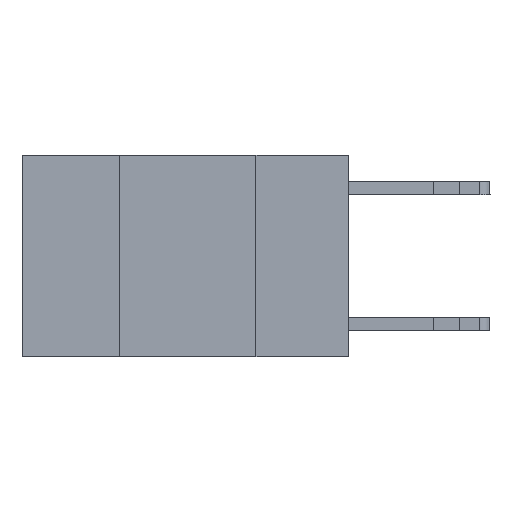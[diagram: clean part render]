
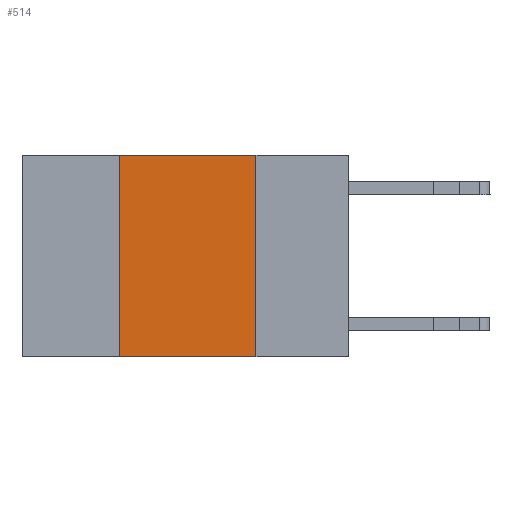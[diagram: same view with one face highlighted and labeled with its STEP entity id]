
A CAD part, left-side view. The second image highlights one B-rep face of the part: STEP entity #514.
In plain terms, the highlighted planar face has unit normal (-1, 0, 0).
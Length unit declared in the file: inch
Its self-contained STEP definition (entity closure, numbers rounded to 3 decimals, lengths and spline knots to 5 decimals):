
#38 = LINE ( 'NONE', #8970, #4514 ) ;
#266 = DIRECTION ( 'NONE',  ( 0., -1., 0. ) ) ;
#419 = EDGE_CURVE ( 'NONE', #13490, #11235, #10476, .T. ) ;
#514 = ADVANCED_FACE ( 'NONE', ( #8455 ), #6282, .F. ) ;
#567 = EDGE_LOOP ( 'NONE', ( #2746, #7116, #1142, #1921 ) ) ;
#623 = CARTESIAN_POINT ( 'NONE',  ( 0., 0.6, -0.37 ) ) ;
#1142 = ORIENTED_EDGE ( 'NONE', *, *, #1852, .F. ) ;
#1598 = AXIS2_PLACEMENT_3D ( 'NONE', #2916, #14141, #8526 ) ;
#1852 = EDGE_CURVE ( 'NONE', #10984, #3160, #9462, .T. ) ;
#1921 = ORIENTED_EDGE ( 'NONE', *, *, #7940, .T. ) ;
#2098 = LINE ( 'NONE', #623, #3636 ) ;
#2198 = CARTESIAN_POINT ( 'NONE',  ( 0., 0.17, 0. ) ) ;
#2746 = ORIENTED_EDGE ( 'NONE', *, *, #419, .F. ) ;
#2916 = CARTESIAN_POINT ( 'NONE',  ( 0., 0.6, 0. ) ) ;
#3160 = VERTEX_POINT ( 'NONE', #5962 ) ;
#3636 = VECTOR ( 'NONE', #4002, 39.37008 ) ;
#4002 = DIRECTION ( 'NONE',  ( 0., -1., 0. ) ) ;
#4081 = DIRECTION ( 'NONE',  ( 0., 0., 1. ) ) ;
#4514 = VECTOR ( 'NONE', #266, 39.37008 ) ;
#5670 = VECTOR ( 'NONE', #4081, 39.37008 ) ;
#5770 = EDGE_CURVE ( 'NONE', #3160, #13490, #38, .T. ) ;
#5962 = CARTESIAN_POINT ( 'NONE',  ( 0., 0.42, 0. ) ) ;
#6042 = CARTESIAN_POINT ( 'NONE',  ( 0., 0.42, -0.37 ) ) ;
#6282 = PLANE ( 'NONE',  #1598 ) ;
#6935 = DIRECTION ( 'NONE',  ( 0., 0., -1. ) ) ;
#7116 = ORIENTED_EDGE ( 'NONE', *, *, #5770, .F. ) ;
#7657 = VECTOR ( 'NONE', #6935, 39.37008 ) ;
#7940 = EDGE_CURVE ( 'NONE', #10984, #11235, #2098, .T. ) ;
#8455 = FACE_OUTER_BOUND ( 'NONE', #567, .T. ) ;
#8526 = DIRECTION ( 'NONE',  ( 0., 0., -1. ) ) ;
#8970 = CARTESIAN_POINT ( 'NONE',  ( 0., 0.6, 0. ) ) ;
#9462 = LINE ( 'NONE', #10839, #5670 ) ;
#10476 = LINE ( 'NONE', #12462, #7657 ) ;
#10839 = CARTESIAN_POINT ( 'NONE',  ( 0., 0.42, 0. ) ) ;
#10984 = VERTEX_POINT ( 'NONE', #6042 ) ;
#11235 = VERTEX_POINT ( 'NONE', #12153 ) ;
#12153 = CARTESIAN_POINT ( 'NONE',  ( 0., 0.17, -0.37 ) ) ;
#12462 = CARTESIAN_POINT ( 'NONE',  ( 0., 0.17, 0. ) ) ;
#13490 = VERTEX_POINT ( 'NONE', #2198 ) ;
#14141 = DIRECTION ( 'NONE',  ( 1., 0., 0. ) ) ;
